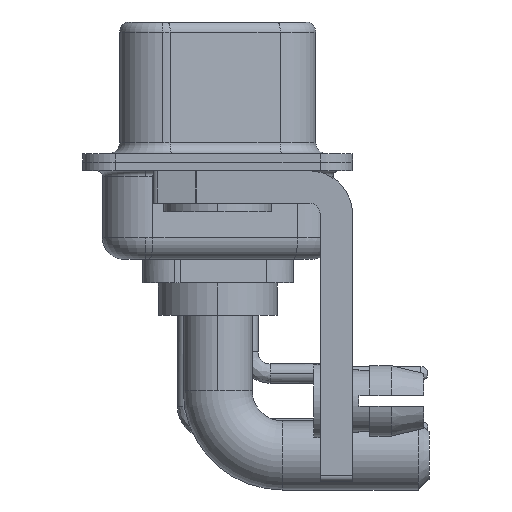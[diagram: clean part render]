
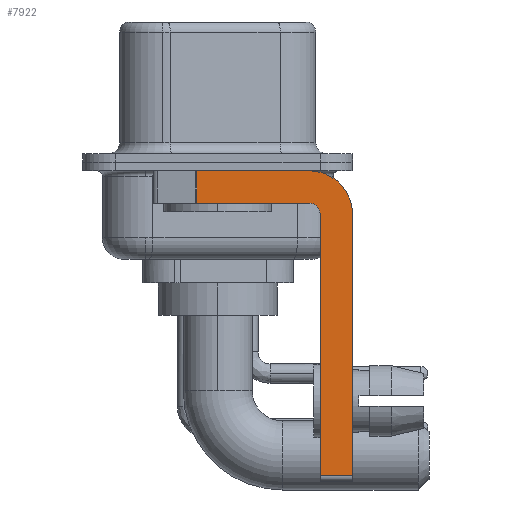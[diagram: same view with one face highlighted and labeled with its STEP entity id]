
A CAD part, left-side view. The second image highlights one B-rep face of the part: STEP entity #7922.
In plain terms, the highlighted planar face has unit normal (-1, 0, 0).
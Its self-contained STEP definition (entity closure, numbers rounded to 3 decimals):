
#14 = DIRECTION ( 'NONE',  ( 1., 0., 0. ) ) ;
#794 = ORIENTED_EDGE ( 'NONE', *, *, #8133, .F. ) ;
#854 = VECTOR ( 'NONE', #20381, 1000. ) ;
#1332 = EDGE_LOOP ( 'NONE', ( #794, #23675, #2655, #10647, #25219, #25813, #5277, #5401 ) ) ;
#1616 = VECTOR ( 'NONE', #3639, 1000. ) ;
#2655 = ORIENTED_EDGE ( 'NONE', *, *, #4929, .F. ) ;
#2812 = VERTEX_POINT ( 'NONE', #25716 ) ;
#3639 = DIRECTION ( 'NONE',  ( 0., 0., 1. ) ) ;
#4086 = DIRECTION ( 'NONE',  ( 0., 0., -1. ) ) ;
#4666 = DIRECTION ( 'NONE',  ( -1., 0., 0. ) ) ;
#4929 = EDGE_CURVE ( 'NONE', #9756, #8923, #22223, .T. ) ;
#5025 = CARTESIAN_POINT ( 'NONE',  ( -2.9, 3., -0.4 ) ) ;
#5277 = ORIENTED_EDGE ( 'NONE', *, *, #23191, .F. ) ;
#5401 = ORIENTED_EDGE ( 'NONE', *, *, #16539, .F. ) ;
#6187 = CARTESIAN_POINT ( 'NONE',  ( -2.9, -4.25, -1.9 ) ) ;
#6982 = LINE ( 'NONE', #5025, #854 ) ;
#7585 = CARTESIAN_POINT ( 'NONE',  ( -2.9, -4.75, -14.8 ) ) ;
#7714 = VERTEX_POINT ( 'NONE', #15035 ) ;
#7799 = CARTESIAN_POINT ( 'NONE',  ( -2.9, -4.25, -1.9 ) ) ;
#7922 = ADVANCED_FACE ( 'NONE', ( #14216 ), #22095, .F. ) ;
#8133 = EDGE_CURVE ( 'NONE', #15676, #7714, #6982, .T. ) ;
#8585 = CARTESIAN_POINT ( 'NONE',  ( -2.9, -4.25, -2.4 ) ) ;
#8749 = VECTOR ( 'NONE', #25796, 1000. ) ;
#8923 = VERTEX_POINT ( 'NONE', #20202 ) ;
#9045 = LINE ( 'NONE', #18767, #13382 ) ;
#9756 = VERTEX_POINT ( 'NONE', #7799 ) ;
#10647 = ORIENTED_EDGE ( 'NONE', *, *, #11535, .F. ) ;
#11535 = EDGE_CURVE ( 'NONE', #21281, #9756, #22798, .T. ) ;
#11815 = EDGE_CURVE ( 'NONE', #15676, #8923, #9045, .T. ) ;
#11926 = DIRECTION ( 'NONE',  ( 0., -1., 0. ) ) ;
#12018 = EDGE_CURVE ( 'NONE', #18479, #21281, #25589, .T. ) ;
#12250 = AXIS2_PLACEMENT_3D ( 'NONE', #25843, #17574, #13900 ) ;
#12388 = LINE ( 'NONE', #17775, #8749 ) ;
#12413 = VERTEX_POINT ( 'NONE', #18134 ) ;
#12665 = CIRCLE ( 'NONE', #12250, 2. ) ;
#13382 = VECTOR ( 'NONE', #17081, 1000. ) ;
#13900 = DIRECTION ( 'NONE',  ( 0., 0., -1. ) ) ;
#13912 = LINE ( 'NONE', #22308, #23638 ) ;
#14087 = DIRECTION ( 'NONE',  ( 0., 1., 0. ) ) ;
#14216 = FACE_OUTER_BOUND ( 'NONE', #1332, .T. ) ;
#14834 = AXIS2_PLACEMENT_3D ( 'NONE', #8585, #4666, #24476 ) ;
#15035 = CARTESIAN_POINT ( 'NONE',  ( -2.9, -4.25, -0.4 ) ) ;
#15676 = VERTEX_POINT ( 'NONE', #22245 ) ;
#15849 = CARTESIAN_POINT ( 'NONE',  ( -2.9, -4.75, -2.4 ) ) ;
#16018 = AXIS2_PLACEMENT_3D ( 'NONE', #18011, #14, #4086 ) ;
#16539 = EDGE_CURVE ( 'NONE', #7714, #12413, #12665, .T. ) ;
#17081 = DIRECTION ( 'NONE',  ( 0., 0., -1. ) ) ;
#17574 = DIRECTION ( 'NONE',  ( 1., 0., 0. ) ) ;
#17775 = CARTESIAN_POINT ( 'NONE',  ( -2.9, -6.25, -2.4 ) ) ;
#18011 = CARTESIAN_POINT ( 'NONE',  ( -2.9, -4.25, -2.4 ) ) ;
#18134 = CARTESIAN_POINT ( 'NONE',  ( -2.9, -6.25, -2.4 ) ) ;
#18479 = VERTEX_POINT ( 'NONE', #22269 ) ;
#18767 = CARTESIAN_POINT ( 'NONE',  ( -2.9, 0.978, -1.9 ) ) ;
#19849 = EDGE_CURVE ( 'NONE', #18479, #2812, #13912, .T. ) ;
#20202 = CARTESIAN_POINT ( 'NONE',  ( -2.9, 0.978, -1.9 ) ) ;
#20381 = DIRECTION ( 'NONE',  ( 0., -1., 0. ) ) ;
#20674 = VECTOR ( 'NONE', #14087, 1000. ) ;
#21281 = VERTEX_POINT ( 'NONE', #15849 ) ;
#22095 = PLANE ( 'NONE',  #16018 ) ;
#22223 = LINE ( 'NONE', #6187, #20674 ) ;
#22245 = CARTESIAN_POINT ( 'NONE',  ( -2.9, 0.978, -0.4 ) ) ;
#22269 = CARTESIAN_POINT ( 'NONE',  ( -2.9, -4.75, -14.55 ) ) ;
#22308 = CARTESIAN_POINT ( 'NONE',  ( -2.9, -4.25, -14.55 ) ) ;
#22798 = CIRCLE ( 'NONE', #14834, 0.5 ) ;
#23191 = EDGE_CURVE ( 'NONE', #12413, #2812, #12388, .T. ) ;
#23638 = VECTOR ( 'NONE', #11926, 1000. ) ;
#23675 = ORIENTED_EDGE ( 'NONE', *, *, #11815, .T. ) ;
#24476 = DIRECTION ( 'NONE',  ( 0., 0., 1. ) ) ;
#25219 = ORIENTED_EDGE ( 'NONE', *, *, #12018, .F. ) ;
#25589 = LINE ( 'NONE', #7585, #1616 ) ;
#25716 = CARTESIAN_POINT ( 'NONE',  ( -2.9, -6.25, -14.55 ) ) ;
#25796 = DIRECTION ( 'NONE',  ( 0., 0., -1. ) ) ;
#25813 = ORIENTED_EDGE ( 'NONE', *, *, #19849, .T. ) ;
#25843 = CARTESIAN_POINT ( 'NONE',  ( -2.9, -4.25, -2.4 ) ) ;
